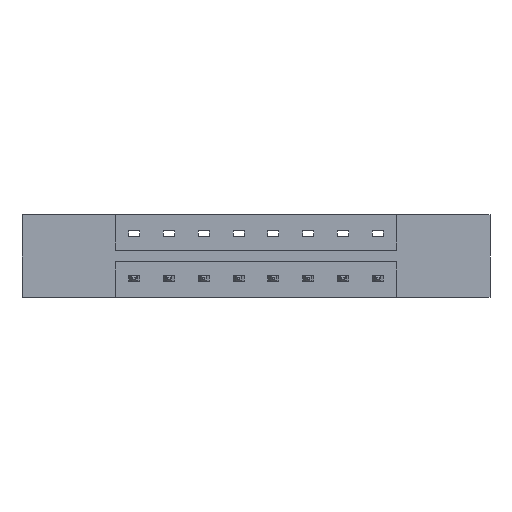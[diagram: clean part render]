
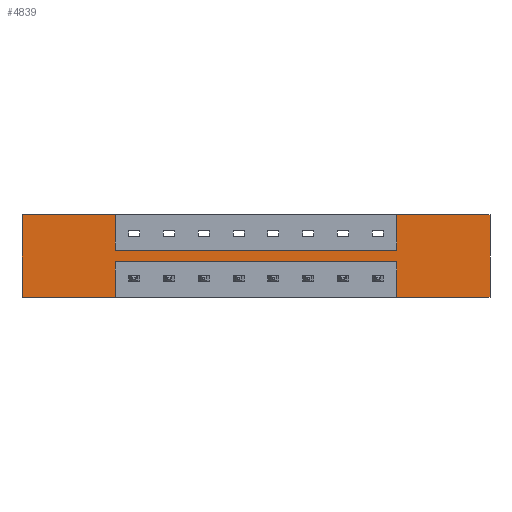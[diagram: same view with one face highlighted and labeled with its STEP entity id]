
A CAD part, front view. The second image highlights one B-rep face of the part: STEP entity #4839.
In plain terms, the highlighted planar face has unit normal (0, -1, 0).
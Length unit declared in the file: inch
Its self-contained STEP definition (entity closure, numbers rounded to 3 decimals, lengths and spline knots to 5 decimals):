
#31 = CARTESIAN_POINT ( 'NONE',  ( 0.4175, 0., -0.1585 ) ) ;
#36 = DIRECTION ( 'NONE',  ( 0., 0., -1. ) ) ;
#135 = LINE ( 'NONE', #2151, #1330 ) ;
#166 = VECTOR ( 'NONE', #3053, 39.37008 ) ;
#184 = ORIENTED_EDGE ( 'NONE', *, *, #8344, .F. ) ;
#351 = EDGE_CURVE ( 'NONE', #9079, #4140, #2032, .T. ) ;
#404 = CARTESIAN_POINT ( 'NONE',  ( 0., 0., -0.37 ) ) ;
#446 = DIRECTION ( 'NONE',  ( 0., -1., 0. ) ) ;
#529 = ORIENTED_EDGE ( 'NONE', *, *, #1441, .F. ) ;
#589 = CARTESIAN_POINT ( 'NONE',  ( 1.6785, 0., -0.1585 ) ) ;
#669 = EDGE_CURVE ( 'NONE', #9053, #4580, #4513, .T. ) ;
#719 = ORIENTED_EDGE ( 'NONE', *, *, #669, .F. ) ;
#777 = LINE ( 'NONE', #3779, #6032 ) ;
#921 = EDGE_LOOP ( 'NONE', ( #1216, #2961, #529, #7309, #1923, #2748, #8021, #7603, #7672, #719, #1349, #184 ) ) ;
#1005 = LINE ( 'NONE', #3063, #5129 ) ;
#1216 = ORIENTED_EDGE ( 'NONE', *, *, #7753, .F. ) ;
#1256 = LINE ( 'NONE', #2614, #5919 ) ;
#1330 = VECTOR ( 'NONE', #36, 39.37008 ) ;
#1349 = ORIENTED_EDGE ( 'NONE', *, *, #3726, .F. ) ;
#1441 = EDGE_CURVE ( 'NONE', #2852, #3678, #135, .T. ) ;
#1473 = CARTESIAN_POINT ( 'NONE',  ( 0.4175, 0., -0.2115 ) ) ;
#1683 = EDGE_CURVE ( 'NONE', #7947, #2852, #4270, .T. ) ;
#1840 = AXIS2_PLACEMENT_3D ( 'NONE', #404, #446, #3257 ) ;
#1893 = FACE_OUTER_BOUND ( 'NONE', #921, .T. ) ;
#1912 = DIRECTION ( 'NONE',  ( 1., 0., 0. ) ) ;
#1923 = ORIENTED_EDGE ( 'NONE', *, *, #7447, .F. ) ;
#1984 = VERTEX_POINT ( 'NONE', #6876 ) ;
#2032 = LINE ( 'NONE', #4909, #7020 ) ;
#2122 = LINE ( 'NONE', #8525, #2557 ) ;
#2150 = CARTESIAN_POINT ( 'NONE',  ( 0.4175, 0., -0.37 ) ) ;
#2151 = CARTESIAN_POINT ( 'NONE',  ( 2.096, 0., 0. ) ) ;
#2255 = CARTESIAN_POINT ( 'NONE',  ( 0.4175, 0., -0.2115 ) ) ;
#2298 = LINE ( 'NONE', #7375, #166 ) ;
#2334 = CARTESIAN_POINT ( 'NONE',  ( 2.096, 0., 0. ) ) ;
#2397 = DIRECTION ( 'NONE',  ( 0., 0., 1. ) ) ;
#2557 = VECTOR ( 'NONE', #3526, 39.37008 ) ;
#2614 = CARTESIAN_POINT ( 'NONE',  ( 0.4175, 0., -0.2115 ) ) ;
#2748 = ORIENTED_EDGE ( 'NONE', *, *, #6931, .F. ) ;
#2754 = DIRECTION ( 'NONE',  ( -1., 0., 0. ) ) ;
#2852 = VERTEX_POINT ( 'NONE', #2334 ) ;
#2961 = ORIENTED_EDGE ( 'NONE', *, *, #6512, .F. ) ;
#2976 = CARTESIAN_POINT ( 'NONE',  ( 0., 0., -0.37 ) ) ;
#3053 = DIRECTION ( 'NONE',  ( 1., 0., 0. ) ) ;
#3063 = CARTESIAN_POINT ( 'NONE',  ( 0., 0., -0.37 ) ) ;
#3122 = CARTESIAN_POINT ( 'NONE',  ( 1.6785, 0., 0. ) ) ;
#3257 = DIRECTION ( 'NONE',  ( 0., 0., -1. ) ) ;
#3526 = DIRECTION ( 'NONE',  ( 1., 0., 0. ) ) ;
#3678 = VERTEX_POINT ( 'NONE', #4592 ) ;
#3726 = EDGE_CURVE ( 'NONE', #4571, #9053, #8710, .T. ) ;
#3779 = CARTESIAN_POINT ( 'NONE',  ( 1.6785, 0., -0.2115 ) ) ;
#3817 = VERTEX_POINT ( 'NONE', #3894 ) ;
#3825 = DIRECTION ( 'NONE',  ( 0., 0., 1. ) ) ;
#3894 = CARTESIAN_POINT ( 'NONE',  ( 1.6785, 0., -0.37 ) ) ;
#3902 = DIRECTION ( 'NONE',  ( -1., 0., 0. ) ) ;
#4072 = VECTOR ( 'NONE', #4688, 39.37008 ) ;
#4140 = VERTEX_POINT ( 'NONE', #31 ) ;
#4270 = LINE ( 'NONE', #9083, #8238 ) ;
#4414 = VERTEX_POINT ( 'NONE', #589 ) ;
#4452 = CARTESIAN_POINT ( 'NONE',  ( 0., 0., 0. ) ) ;
#4513 = LINE ( 'NONE', #4659, #8873 ) ;
#4571 = VERTEX_POINT ( 'NONE', #1473 ) ;
#4580 = VERTEX_POINT ( 'NONE', #2976 ) ;
#4592 = CARTESIAN_POINT ( 'NONE',  ( 2.096, 0., -0.37 ) ) ;
#4659 = CARTESIAN_POINT ( 'NONE',  ( 0., 0., -0.37 ) ) ;
#4688 = DIRECTION ( 'NONE',  ( 0., 0., 1. ) ) ;
#4839 = ADVANCED_FACE ( 'NONE', ( #1893 ), #6925, .T. ) ;
#4909 = CARTESIAN_POINT ( 'NONE',  ( 0.4175, 0., -0.1585 ) ) ;
#5128 = DIRECTION ( 'NONE',  ( 0., 0., -1. ) ) ;
#5129 = VECTOR ( 'NONE', #6592, 39.37008 ) ;
#5221 = VERTEX_POINT ( 'NONE', #8317 ) ;
#5615 = DIRECTION ( 'NONE',  ( 0., 0., -1. ) ) ;
#5919 = VECTOR ( 'NONE', #2754, 39.37008 ) ;
#6032 = VECTOR ( 'NONE', #3825, 39.37008 ) ;
#6289 = CARTESIAN_POINT ( 'NONE',  ( 0.4175, 0., 0. ) ) ;
#6349 = EDGE_CURVE ( 'NONE', #1984, #9079, #2122, .T. ) ;
#6512 = EDGE_CURVE ( 'NONE', #3678, #3817, #1005, .T. ) ;
#6592 = DIRECTION ( 'NONE',  ( -1., 0., 0. ) ) ;
#6766 = VECTOR ( 'NONE', #5128, 39.37008 ) ;
#6876 = CARTESIAN_POINT ( 'NONE',  ( 0., 0., 0. ) ) ;
#6925 = PLANE ( 'NONE',  #1840 ) ;
#6931 = EDGE_CURVE ( 'NONE', #4140, #4414, #2298, .T. ) ;
#7020 = VECTOR ( 'NONE', #5615, 39.37008 ) ;
#7309 = ORIENTED_EDGE ( 'NONE', *, *, #1683, .F. ) ;
#7375 = CARTESIAN_POINT ( 'NONE',  ( 0.4175, 0., -0.1585 ) ) ;
#7447 = EDGE_CURVE ( 'NONE', #4414, #7947, #8979, .T. ) ;
#7598 = CARTESIAN_POINT ( 'NONE',  ( 1.6785, 0., -0.1585 ) ) ;
#7603 = ORIENTED_EDGE ( 'NONE', *, *, #6349, .F. ) ;
#7672 = ORIENTED_EDGE ( 'NONE', *, *, #8302, .F. ) ;
#7753 = EDGE_CURVE ( 'NONE', #3817, #5221, #777, .T. ) ;
#7947 = VERTEX_POINT ( 'NONE', #3122 ) ;
#7984 = VECTOR ( 'NONE', #2397, 39.37008 ) ;
#8021 = ORIENTED_EDGE ( 'NONE', *, *, #351, .F. ) ;
#8238 = VECTOR ( 'NONE', #1912, 39.37008 ) ;
#8302 = EDGE_CURVE ( 'NONE', #4580, #1984, #8849, .T. ) ;
#8317 = CARTESIAN_POINT ( 'NONE',  ( 1.6785, 0., -0.2115 ) ) ;
#8344 = EDGE_CURVE ( 'NONE', #5221, #4571, #1256, .T. ) ;
#8525 = CARTESIAN_POINT ( 'NONE',  ( 0., 0., 0. ) ) ;
#8710 = LINE ( 'NONE', #2255, #6766 ) ;
#8849 = LINE ( 'NONE', #4452, #7984 ) ;
#8873 = VECTOR ( 'NONE', #3902, 39.37008 ) ;
#8979 = LINE ( 'NONE', #7598, #4072 ) ;
#9053 = VERTEX_POINT ( 'NONE', #2150 ) ;
#9079 = VERTEX_POINT ( 'NONE', #6289 ) ;
#9083 = CARTESIAN_POINT ( 'NONE',  ( 0., 0., 0. ) ) ;
